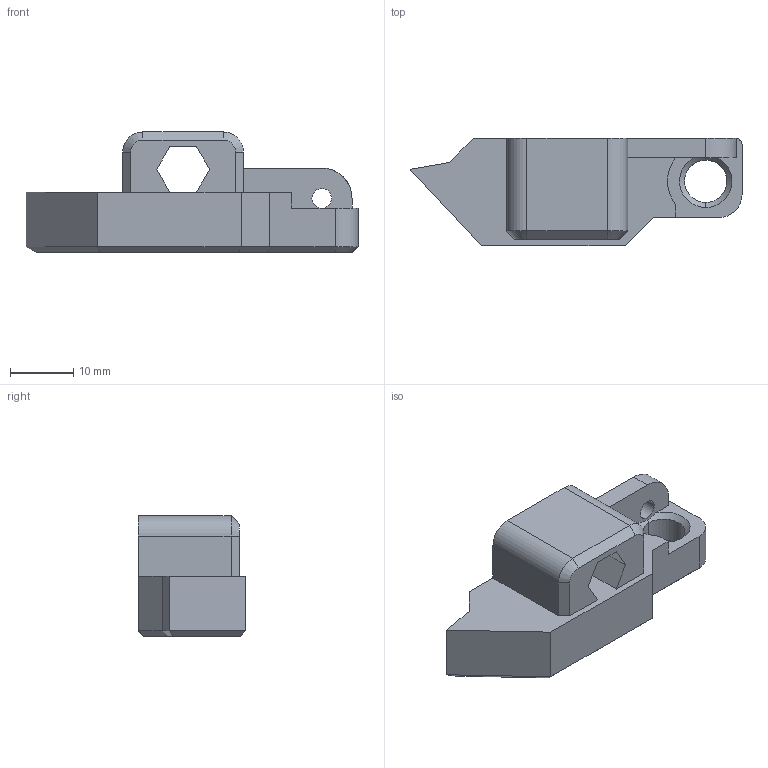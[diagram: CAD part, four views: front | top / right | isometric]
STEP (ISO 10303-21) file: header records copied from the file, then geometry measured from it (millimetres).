
FILE_DESCRIPTION (( 'STEP AP203' ), '1' );
FILE_NAME ('AF-HF-LR-PRT-004-STEP.STEP', '2020-11-05T06:55:17', ( '' ), ( '' ), 'SwSTEP 2.0', 'SolidWorks 2018', '' );
FILE_SCHEMA (( 'CONFIG_CONTROL_DESIGN' ));
Length unit declared in the file: inch
Products named in the file (1): AF-HF-LR-PRT-004-STEP
Bounding box: 52.35 x 16.89 x 18.94 mm (x, y, z)
Volume: 6709.3 mm3; surface area: 4395.1 mm2
Topology: 1 solids, 1 shells, 129 faces, 335 edges, 208 vertices
Faces by surface type: plane 73, cylinder 39, cone 11, bspline 6
Entity records: 5335 total; most frequent: CARTESIAN_POINT 2204, ORIENTED_EDGE 670, DIRECTION 600, EDGE_CURVE 335, LINE 228, VECTOR 228, VERTEX_POINT 208, AXIS2_PLACEMENT_3D 186
